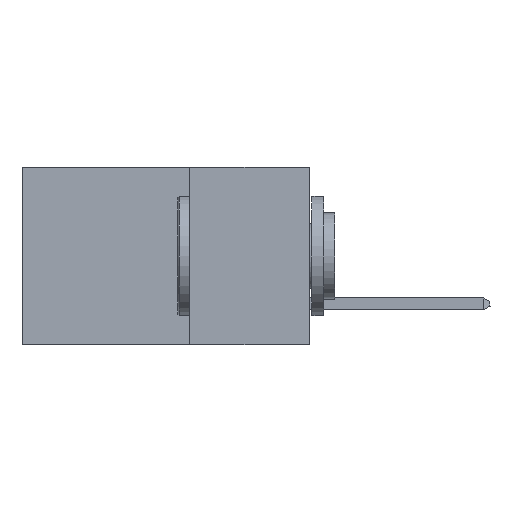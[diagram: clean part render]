
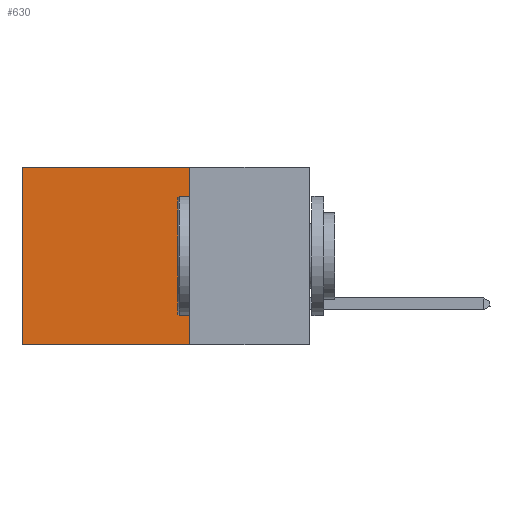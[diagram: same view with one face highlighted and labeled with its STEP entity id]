
A CAD part, left-side view. The second image highlights one B-rep face of the part: STEP entity #630.
In plain terms, the highlighted planar face has unit normal (-1, 0, 0).
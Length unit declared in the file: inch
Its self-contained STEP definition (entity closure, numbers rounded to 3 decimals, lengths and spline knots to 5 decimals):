
#96 = EDGE_CURVE ( 'NONE', #20412, #19719, #29932, .T. ) ;
#630 = ADVANCED_FACE ( 'NONE', ( #1917 ), #15126, .F. ) ;
#1140 = DIRECTION ( 'NONE',  ( 0., 0., -1. ) ) ;
#1772 = VECTOR ( 'NONE', #15097, 39.37008 ) ;
#1917 = FACE_OUTER_BOUND ( 'NONE', #32256, .T. ) ;
#3926 = EDGE_CURVE ( 'NONE', #26395, #19747, #25903, .T. ) ;
#5048 = ORIENTED_EDGE ( 'NONE', *, *, #30431, .T. ) ;
#6620 = VECTOR ( 'NONE', #13793, 39.37008 ) ;
#10153 = CARTESIAN_POINT ( 'NONE',  ( 0.2875, 0.6, 0. ) ) ;
#10364 = CARTESIAN_POINT ( 'NONE',  ( 0.2875, 0.6, 0. ) ) ;
#12559 = CARTESIAN_POINT ( 'NONE',  ( 0.2875, 0.25, -0.37 ) ) ;
#13107 = ORIENTED_EDGE ( 'NONE', *, *, #37082, .F. ) ;
#13454 = ORIENTED_EDGE ( 'NONE', *, *, #3926, .T. ) ;
#13740 = VECTOR ( 'NONE', #25616, 39.37008 ) ;
#13793 = DIRECTION ( 'NONE',  ( 0., 0., -1. ) ) ;
#14571 = LINE ( 'NONE', #32015, #6620 ) ;
#15049 = CARTESIAN_POINT ( 'NONE',  ( 0.2875, 0.25, 0. ) ) ;
#15097 = DIRECTION ( 'NONE',  ( 0., 1., 0. ) ) ;
#15126 = PLANE ( 'NONE',  #23669 ) ;
#18190 = DIRECTION ( 'NONE',  ( 0., 0., -1. ) ) ;
#19719 = VERTEX_POINT ( 'NONE', #22222 ) ;
#19747 = VERTEX_POINT ( 'NONE', #10364 ) ;
#20412 = VERTEX_POINT ( 'NONE', #31638 ) ;
#22222 = CARTESIAN_POINT ( 'NONE',  ( 0.2875, 0.6, -0.37 ) ) ;
#23070 = VECTOR ( 'NONE', #1140, 39.37008 ) ;
#23669 = AXIS2_PLACEMENT_3D ( 'NONE', #39100, #36343, #18190 ) ;
#25616 = DIRECTION ( 'NONE',  ( 0., 1., 0. ) ) ;
#25903 = LINE ( 'NONE', #30290, #1772 ) ;
#26395 = VERTEX_POINT ( 'NONE', #15049 ) ;
#27044 = ORIENTED_EDGE ( 'NONE', *, *, #96, .F. ) ;
#29932 = LINE ( 'NONE', #12559, #13740 ) ;
#30290 = CARTESIAN_POINT ( 'NONE',  ( 0.2875, 0.25, 0. ) ) ;
#30431 = EDGE_CURVE ( 'NONE', #19747, #19719, #32159, .T. ) ;
#31638 = CARTESIAN_POINT ( 'NONE',  ( 0.2875, 0.25, -0.37 ) ) ;
#32015 = CARTESIAN_POINT ( 'NONE',  ( 0.2875, 0.25, 0. ) ) ;
#32159 = LINE ( 'NONE', #10153, #23070 ) ;
#32256 = EDGE_LOOP ( 'NONE', ( #5048, #27044, #13107, #13454 ) ) ;
#36343 = DIRECTION ( 'NONE',  ( 1., 0., 0. ) ) ;
#37082 = EDGE_CURVE ( 'NONE', #26395, #20412, #14571, .T. ) ;
#39100 = CARTESIAN_POINT ( 'NONE',  ( 0.2875, 0.25, 0. ) ) ;
